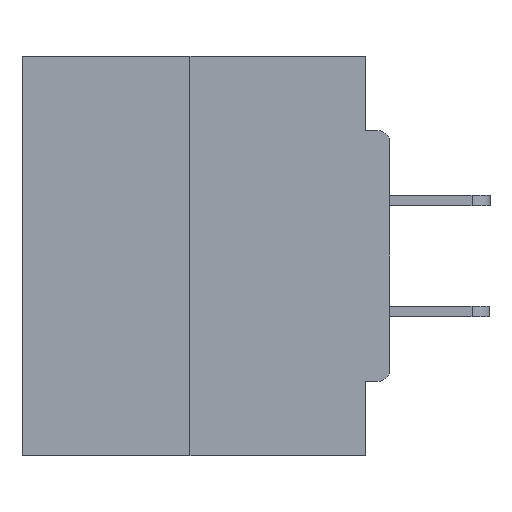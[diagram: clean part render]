
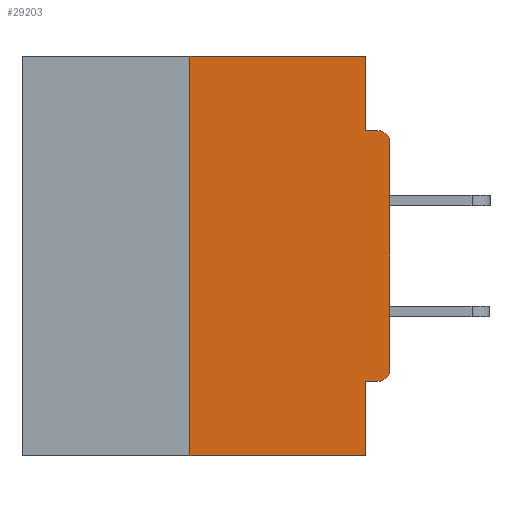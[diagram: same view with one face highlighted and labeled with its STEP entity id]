
A CAD part, left-side view. The second image highlights one B-rep face of the part: STEP entity #29203.
In plain terms, the highlighted planar face has unit normal (-1, 0, 0).
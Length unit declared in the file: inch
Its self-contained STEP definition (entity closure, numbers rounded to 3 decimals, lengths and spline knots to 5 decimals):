
#752 = VERTEX_POINT ( 'NONE', #35653 ) ;
#885 = LINE ( 'NONE', #23465, #31965 ) ;
#1575 = EDGE_CURVE ( 'NONE', #12004, #752, #16408, .T. ) ;
#1586 = ORIENTED_EDGE ( 'NONE', *, *, #39609, .F. ) ;
#2179 = AXIS2_PLACEMENT_3D ( 'NONE', #24234, #20629, #27686 ) ;
#3004 = EDGE_CURVE ( 'NONE', #19371, #752, #3710, .T. ) ;
#3009 = DIRECTION ( 'NONE',  ( 0., 0., 1. ) ) ;
#3677 = DIRECTION ( 'NONE',  ( -1., 0., 0. ) ) ;
#3710 = CIRCLE ( 'NONE', #2179, 0.015 ) ;
#3932 = ORIENTED_EDGE ( 'NONE', *, *, #3004, .T. ) ;
#3943 = DIRECTION ( 'NONE',  ( 0., 0., -1. ) ) ;
#4436 = ORIENTED_EDGE ( 'NONE', *, *, #22493, .T. ) ;
#5285 = CARTESIAN_POINT ( 'NONE',  ( 0., 0.031, 0. ) ) ;
#5805 = LINE ( 'NONE', #20272, #40056 ) ;
#7844 = PLANE ( 'NONE',  #16958 ) ;
#11066 = CARTESIAN_POINT ( 'NONE',  ( 0., 0.46, -0.5 ) ) ;
#11076 = EDGE_CURVE ( 'NONE', #32939, #32443, #19321, .T. ) ;
#11873 = EDGE_CURVE ( 'NONE', #17319, #20905, #21943, .T. ) ;
#11950 = CARTESIAN_POINT ( 'NONE',  ( 0., 0., -0.0935 ) ) ;
#12004 = VERTEX_POINT ( 'NONE', #21679 ) ;
#12913 = CARTESIAN_POINT ( 'NONE',  ( 0., 0.031, -0.5 ) ) ;
#13153 = CARTESIAN_POINT ( 'NONE',  ( 0., 0., 0. ) ) ;
#13274 = CARTESIAN_POINT ( 'NONE',  ( 0., 0.25, -0.5 ) ) ;
#13292 = VECTOR ( 'NONE', #17974, 39.37008 ) ;
#13530 = DIRECTION ( 'NONE',  ( 0., -1., 0. ) ) ;
#14448 = ORIENTED_EDGE ( 'NONE', *, *, #40257, .T. ) ;
#14471 = DIRECTION ( 'NONE',  ( 0., -1., 0. ) ) ;
#15019 = EDGE_LOOP ( 'NONE', ( #1586, #29556, #4436, #19316, #21074, #22563, #14448, #3932, #41739, #33467 ) ) ;
#15412 = LINE ( 'NONE', #17830, #13292 ) ;
#15893 = VERTEX_POINT ( 'NONE', #24613 ) ;
#16114 = AXIS2_PLACEMENT_3D ( 'NONE', #20668, #3677, #23842 ) ;
#16408 = LINE ( 'NONE', #11950, #21260 ) ;
#16958 = AXIS2_PLACEMENT_3D ( 'NONE', #18049, #42117, #3943 ) ;
#17319 = VERTEX_POINT ( 'NONE', #23841 ) ;
#17521 = VECTOR ( 'NONE', #14471, 39.37008 ) ;
#17830 = CARTESIAN_POINT ( 'NONE',  ( 0., 0., -0.4065 ) ) ;
#17974 = DIRECTION ( 'NONE',  ( 0., 1., 0. ) ) ;
#18049 = CARTESIAN_POINT ( 'NONE',  ( 0., 0.46, 0. ) ) ;
#18481 = DIRECTION ( 'NONE',  ( 0., -1., 0. ) ) ;
#19316 = ORIENTED_EDGE ( 'NONE', *, *, #11873, .F. ) ;
#19321 = CIRCLE ( 'NONE', #16114, 0.015 ) ;
#19371 = VERTEX_POINT ( 'NONE', #24630 ) ;
#20272 = CARTESIAN_POINT ( 'NONE',  ( 0., 0.46, 0. ) ) ;
#20629 = DIRECTION ( 'NONE',  ( -1., 0., 0. ) ) ;
#20668 = CARTESIAN_POINT ( 'NONE',  ( 0., 0.015, -0.3915 ) ) ;
#20905 = VERTEX_POINT ( 'NONE', #12913 ) ;
#21074 = ORIENTED_EDGE ( 'NONE', *, *, #43118, .F. ) ;
#21260 = VECTOR ( 'NONE', #18481, 39.37008 ) ;
#21679 = CARTESIAN_POINT ( 'NONE',  ( 0., 0.031, -0.0935 ) ) ;
#21943 = LINE ( 'NONE', #37152, #23583 ) ;
#22493 = EDGE_CURVE ( 'NONE', #27440, #20905, #28307, .T. ) ;
#22563 = ORIENTED_EDGE ( 'NONE', *, *, #11076, .T. ) ;
#23465 = CARTESIAN_POINT ( 'NONE',  ( 0., 0.25, 0. ) ) ;
#23500 = DIRECTION ( 'NONE',  ( 0., 0., -1. ) ) ;
#23583 = VECTOR ( 'NONE', #23500, 39.37008 ) ;
#23841 = CARTESIAN_POINT ( 'NONE',  ( 0., 0.031, -0.4065 ) ) ;
#23842 = DIRECTION ( 'NONE',  ( 0., 0., -1. ) ) ;
#24234 = CARTESIAN_POINT ( 'NONE',  ( 0., 0.015, -0.1085 ) ) ;
#24613 = CARTESIAN_POINT ( 'NONE',  ( 0., 0.25, 0. ) ) ;
#24630 = CARTESIAN_POINT ( 'NONE',  ( 0., 0., -0.1085 ) ) ;
#25473 = EDGE_CURVE ( 'NONE', #37412, #12004, #29111, .T. ) ;
#26739 = CARTESIAN_POINT ( 'NONE',  ( 0., 0.015, -0.4065 ) ) ;
#27440 = VERTEX_POINT ( 'NONE', #13274 ) ;
#27686 = DIRECTION ( 'NONE',  ( 0., 0., -1. ) ) ;
#28307 = LINE ( 'NONE', #11066, #17521 ) ;
#29111 = LINE ( 'NONE', #36067, #34466 ) ;
#29203 = ADVANCED_FACE ( 'NONE', ( #41617 ), #7844, .F. ) ;
#29402 = EDGE_CURVE ( 'NONE', #27440, #15893, #885, .T. ) ;
#29556 = ORIENTED_EDGE ( 'NONE', *, *, #29402, .F. ) ;
#31965 = VECTOR ( 'NONE', #3009, 39.37008 ) ;
#32322 = DIRECTION ( 'NONE',  ( 0., 0., -1. ) ) ;
#32443 = VERTEX_POINT ( 'NONE', #37076 ) ;
#32939 = VERTEX_POINT ( 'NONE', #26739 ) ;
#33467 = ORIENTED_EDGE ( 'NONE', *, *, #25473, .F. ) ;
#34466 = VECTOR ( 'NONE', #32322, 39.37008 ) ;
#35653 = CARTESIAN_POINT ( 'NONE',  ( 0., 0.015, -0.0935 ) ) ;
#36067 = CARTESIAN_POINT ( 'NONE',  ( 0., 0.031, 0. ) ) ;
#36693 = DIRECTION ( 'NONE',  ( 0., 0., 1. ) ) ;
#37076 = CARTESIAN_POINT ( 'NONE',  ( 0., 0., -0.3915 ) ) ;
#37152 = CARTESIAN_POINT ( 'NONE',  ( 0., 0.031, -0.5 ) ) ;
#37317 = VECTOR ( 'NONE', #36693, 39.37008 ) ;
#37412 = VERTEX_POINT ( 'NONE', #5285 ) ;
#38367 = LINE ( 'NONE', #13153, #37317 ) ;
#39609 = EDGE_CURVE ( 'NONE', #15893, #37412, #5805, .T. ) ;
#40056 = VECTOR ( 'NONE', #13530, 39.37008 ) ;
#40257 = EDGE_CURVE ( 'NONE', #32443, #19371, #38367, .T. ) ;
#41617 = FACE_OUTER_BOUND ( 'NONE', #15019, .T. ) ;
#41739 = ORIENTED_EDGE ( 'NONE', *, *, #1575, .F. ) ;
#42117 = DIRECTION ( 'NONE',  ( 1., 0., 0. ) ) ;
#43118 = EDGE_CURVE ( 'NONE', #32939, #17319, #15412, .T. ) ;
